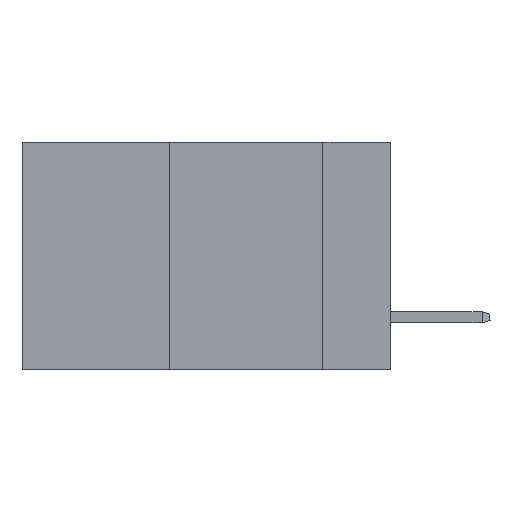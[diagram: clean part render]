
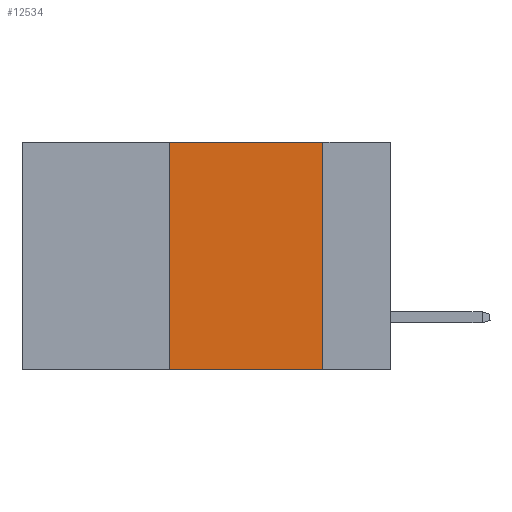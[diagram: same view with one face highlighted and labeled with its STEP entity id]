
A CAD part, left-side view. The second image highlights one B-rep face of the part: STEP entity #12534.
In plain terms, the highlighted planar face has unit normal (-1, 0, 0).
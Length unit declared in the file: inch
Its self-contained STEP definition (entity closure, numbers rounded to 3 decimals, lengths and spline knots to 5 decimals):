
#2997 = CARTESIAN_POINT ( 'NONE',  ( 0., 0.36, 0. ) ) ;
#3958 = VECTOR ( 'NONE', #10635, 39.37008 ) ;
#4106 = CARTESIAN_POINT ( 'NONE',  ( 0., 0.6, 0. ) ) ;
#6151 = DIRECTION ( 'NONE',  ( 0., -1., 0. ) ) ;
#6187 = VERTEX_POINT ( 'NONE', #20565 ) ;
#7649 = DIRECTION ( 'NONE',  ( 0., 0., -1. ) ) ;
#8210 = PLANE ( 'NONE',  #10653 ) ;
#8414 = CARTESIAN_POINT ( 'NONE',  ( 0., 0.6, -0.37 ) ) ;
#8744 = ORIENTED_EDGE ( 'NONE', *, *, #14211, .F. ) ;
#8919 = LINE ( 'NONE', #9955, #18910 ) ;
#8952 = DIRECTION ( 'NONE',  ( 0., 0., -1. ) ) ;
#9029 = DIRECTION ( 'NONE',  ( 0., -1., 0. ) ) ;
#9955 = CARTESIAN_POINT ( 'NONE',  ( 0., 0.11, 0. ) ) ;
#10635 = DIRECTION ( 'NONE',  ( 0., 0., 1. ) ) ;
#10653 = AXIS2_PLACEMENT_3D ( 'NONE', #23953, #17555, #8952 ) ;
#12364 = CARTESIAN_POINT ( 'NONE',  ( 0., 0.36, -0.37 ) ) ;
#12534 = ADVANCED_FACE ( 'NONE', ( #13713 ), #8210, .F. ) ;
#12781 = EDGE_CURVE ( 'NONE', #21554, #6187, #16962, .T. ) ;
#13070 = ORIENTED_EDGE ( 'NONE', *, *, #12781, .T. ) ;
#13713 = FACE_OUTER_BOUND ( 'NONE', #22552, .T. ) ;
#14211 = EDGE_CURVE ( 'NONE', #21554, #19468, #25257, .T. ) ;
#14352 = VECTOR ( 'NONE', #9029, 39.37008 ) ;
#14421 = EDGE_CURVE ( 'NONE', #16532, #6187, #8919, .T. ) ;
#14913 = ORIENTED_EDGE ( 'NONE', *, *, #15117, .F. ) ;
#15117 = EDGE_CURVE ( 'NONE', #19468, #16532, #16126, .T. ) ;
#16126 = LINE ( 'NONE', #4106, #22154 ) ;
#16532 = VERTEX_POINT ( 'NONE', #20083 ) ;
#16962 = LINE ( 'NONE', #8414, #14352 ) ;
#17555 = DIRECTION ( 'NONE',  ( 1., 0., 0. ) ) ;
#18910 = VECTOR ( 'NONE', #7649, 39.37008 ) ;
#19468 = VERTEX_POINT ( 'NONE', #2997 ) ;
#20083 = CARTESIAN_POINT ( 'NONE',  ( 0., 0.11, 0. ) ) ;
#20565 = CARTESIAN_POINT ( 'NONE',  ( 0., 0.11, -0.37 ) ) ;
#21050 = ORIENTED_EDGE ( 'NONE', *, *, #14421, .F. ) ;
#21512 = CARTESIAN_POINT ( 'NONE',  ( 0., 0.36, 0. ) ) ;
#21554 = VERTEX_POINT ( 'NONE', #12364 ) ;
#22154 = VECTOR ( 'NONE', #6151, 39.37008 ) ;
#22552 = EDGE_LOOP ( 'NONE', ( #21050, #14913, #8744, #13070 ) ) ;
#23953 = CARTESIAN_POINT ( 'NONE',  ( 0., 0.6, 0. ) ) ;
#25257 = LINE ( 'NONE', #21512, #3958 ) ;
